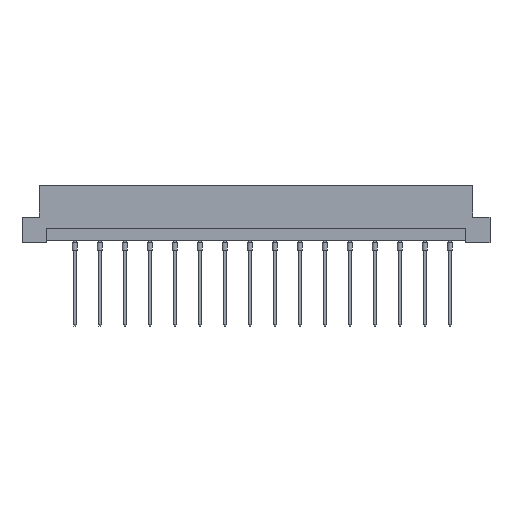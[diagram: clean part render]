
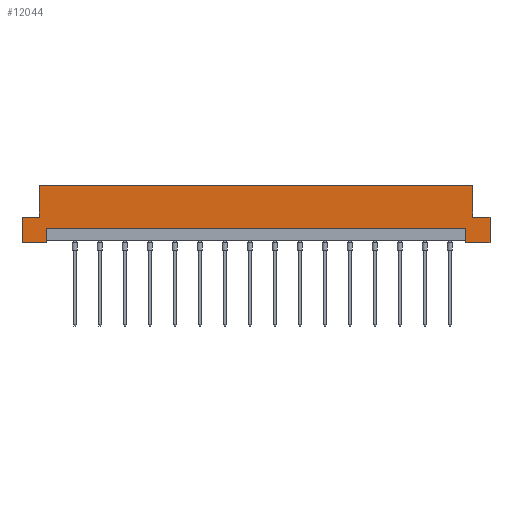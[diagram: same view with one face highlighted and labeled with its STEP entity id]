
A CAD part, front view. The second image highlights one B-rep face of the part: STEP entity #12044.
In plain terms, the highlighted planar face has unit normal (0, -1, 0).
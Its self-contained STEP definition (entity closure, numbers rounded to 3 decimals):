
#254 = LINE ( 'NONE', #3026, #791 ) ;
#526 = EDGE_CURVE ( 'NONE', #8135, #6141, #4010, .T. ) ;
#589 = CARTESIAN_POINT ( 'NONE',  ( -47.5, 0., 5.2 ) ) ;
#791 = VECTOR ( 'NONE', #2764, 1000. ) ;
#903 = LINE ( 'NONE', #14493, #12254 ) ;
#1053 = VECTOR ( 'NONE', #10106, 1000. ) ;
#1087 = VECTOR ( 'NONE', #8696, 1000. ) ;
#1603 = FACE_OUTER_BOUND ( 'NONE', #7244, .T. ) ;
#1693 = DIRECTION ( 'NONE',  ( 0., 1., 0. ) ) ;
#1768 = DIRECTION ( 'NONE',  ( 0., 0., 1. ) ) ;
#1848 = ORIENTED_EDGE ( 'NONE', *, *, #2364, .F. ) ;
#2083 = ORIENTED_EDGE ( 'NONE', *, *, #16746, .T. ) ;
#2117 = VERTEX_POINT ( 'NONE', #13574 ) ;
#2306 = CARTESIAN_POINT ( 'NONE',  ( 47.5, 0., 5.2 ) ) ;
#2364 = EDGE_CURVE ( 'NONE', #9708, #5236, #4027, .T. ) ;
#2464 = CARTESIAN_POINT ( 'NONE',  ( -47.5, 0., 0. ) ) ;
#2494 = VECTOR ( 'NONE', #13591, 1000. ) ;
#2764 = DIRECTION ( 'NONE',  ( -1., 0., 0. ) ) ;
#2993 = DIRECTION ( 'NONE',  ( -1., 0., 0. ) ) ;
#3026 = CARTESIAN_POINT ( 'NONE',  ( 42.6, 0., 2.9 ) ) ;
#3185 = CARTESIAN_POINT ( 'NONE',  ( -44., 0., 11.6 ) ) ;
#3362 = LINE ( 'NONE', #589, #1053 ) ;
#3499 = VERTEX_POINT ( 'NONE', #12302 ) ;
#3605 = EDGE_CURVE ( 'NONE', #7947, #10979, #9857, .T. ) ;
#3827 = VERTEX_POINT ( 'NONE', #9080 ) ;
#3889 = ORIENTED_EDGE ( 'NONE', *, *, #5770, .F. ) ;
#3934 = CARTESIAN_POINT ( 'NONE',  ( -44., 0., 5.2 ) ) ;
#3948 = DIRECTION ( 'NONE',  ( 0., 0., 1. ) ) ;
#4010 = LINE ( 'NONE', #9472, #17035 ) ;
#4027 = LINE ( 'NONE', #2464, #13573 ) ;
#4116 = ORIENTED_EDGE ( 'NONE', *, *, #3605, .F. ) ;
#4282 = CARTESIAN_POINT ( 'NONE',  ( 42.6, 0., 2.9 ) ) ;
#4294 = PLANE ( 'NONE',  #6593 ) ;
#4607 = VERTEX_POINT ( 'NONE', #7876 ) ;
#4753 = DIRECTION ( 'NONE',  ( 0., 0., 1. ) ) ;
#4862 = VECTOR ( 'NONE', #4753, 1000. ) ;
#5236 = VERTEX_POINT ( 'NONE', #9432 ) ;
#5342 = LINE ( 'NONE', #2306, #16268 ) ;
#5584 = ORIENTED_EDGE ( 'NONE', *, *, #7780, .F. ) ;
#5752 = VECTOR ( 'NONE', #13135, 1000. ) ;
#5770 = EDGE_CURVE ( 'NONE', #7161, #11679, #8915, .T. ) ;
#6141 = VERTEX_POINT ( 'NONE', #16254 ) ;
#6461 = CARTESIAN_POINT ( 'NONE',  ( -42.6, 0., 2.9 ) ) ;
#6593 = AXIS2_PLACEMENT_3D ( 'NONE', #13557, #1693, #1768 ) ;
#6619 = VECTOR ( 'NONE', #16775, 1000. ) ;
#6741 = VECTOR ( 'NONE', #2993, 1000. ) ;
#6823 = ORIENTED_EDGE ( 'NONE', *, *, #11260, .F. ) ;
#7161 = VERTEX_POINT ( 'NONE', #6461 ) ;
#7244 = EDGE_LOOP ( 'NONE', ( #14035, #13703, #5584, #14961, #6823, #2083, #13695, #4116, #14685, #1848, #13256, #3889 ) ) ;
#7431 = CARTESIAN_POINT ( 'NONE',  ( -42.6, 0., 0.5 ) ) ;
#7780 = EDGE_CURVE ( 'NONE', #4607, #6141, #12272, .T. ) ;
#7876 = CARTESIAN_POINT ( 'NONE',  ( 47.5, 0., 0. ) ) ;
#7947 = VERTEX_POINT ( 'NONE', #3934 ) ;
#8135 = VERTEX_POINT ( 'NONE', #4282 ) ;
#8140 = LINE ( 'NONE', #11959, #2494 ) ;
#8696 = DIRECTION ( 'NONE',  ( 1., 0., 0. ) ) ;
#8915 = LINE ( 'NONE', #7431, #6619 ) ;
#9080 = CARTESIAN_POINT ( 'NONE',  ( 47.5, 0., 5.2 ) ) ;
#9081 = LINE ( 'NONE', #13057, #5752 ) ;
#9215 = EDGE_CURVE ( 'NONE', #10979, #2117, #12779, .T. ) ;
#9291 = DIRECTION ( 'NONE',  ( 0., 0., -1. ) ) ;
#9432 = CARTESIAN_POINT ( 'NONE',  ( -47.5, 0., 5.2 ) ) ;
#9472 = CARTESIAN_POINT ( 'NONE',  ( 42.6, 0., 0.5 ) ) ;
#9631 = EDGE_CURVE ( 'NONE', #8135, #7161, #254, .T. ) ;
#9708 = VERTEX_POINT ( 'NONE', #10747 ) ;
#9848 = EDGE_CURVE ( 'NONE', #5236, #7947, #3362, .T. ) ;
#9857 = LINE ( 'NONE', #16609, #4862 ) ;
#10106 = DIRECTION ( 'NONE',  ( 1., 0., 0. ) ) ;
#10369 = DIRECTION ( 'NONE',  ( 1., 0., 0. ) ) ;
#10747 = CARTESIAN_POINT ( 'NONE',  ( -47.5, 0., 0. ) ) ;
#10979 = VERTEX_POINT ( 'NONE', #3185 ) ;
#11260 = EDGE_CURVE ( 'NONE', #3499, #3827, #5342, .T. ) ;
#11298 = EDGE_CURVE ( 'NONE', #3827, #4607, #9081, .T. ) ;
#11483 = CARTESIAN_POINT ( 'NONE',  ( -47.5, 0., 11.6 ) ) ;
#11679 = VERTEX_POINT ( 'NONE', #12535 ) ;
#11959 = CARTESIAN_POINT ( 'NONE',  ( -47.5, 0., 0. ) ) ;
#12044 = ADVANCED_FACE ( 'NONE', ( #1603 ), #4294, .F. ) ;
#12254 = VECTOR ( 'NONE', #14153, 1000. ) ;
#12272 = LINE ( 'NONE', #14851, #6741 ) ;
#12302 = CARTESIAN_POINT ( 'NONE',  ( 44., 0., 5.2 ) ) ;
#12535 = CARTESIAN_POINT ( 'NONE',  ( -42.6, 0., 0. ) ) ;
#12779 = LINE ( 'NONE', #11483, #1087 ) ;
#13057 = CARTESIAN_POINT ( 'NONE',  ( 47.5, 0., 0. ) ) ;
#13135 = DIRECTION ( 'NONE',  ( 0., 0., -1. ) ) ;
#13256 = ORIENTED_EDGE ( 'NONE', *, *, #14682, .F. ) ;
#13557 = CARTESIAN_POINT ( 'NONE',  ( -47.5, 0., 11.6 ) ) ;
#13573 = VECTOR ( 'NONE', #3948, 1000. ) ;
#13574 = CARTESIAN_POINT ( 'NONE',  ( 44., 0., 11.6 ) ) ;
#13591 = DIRECTION ( 'NONE',  ( -1., 0., 0. ) ) ;
#13695 = ORIENTED_EDGE ( 'NONE', *, *, #9215, .F. ) ;
#13703 = ORIENTED_EDGE ( 'NONE', *, *, #526, .T. ) ;
#14035 = ORIENTED_EDGE ( 'NONE', *, *, #9631, .F. ) ;
#14153 = DIRECTION ( 'NONE',  ( 0., 0., 1. ) ) ;
#14493 = CARTESIAN_POINT ( 'NONE',  ( 44., 0., 5.2 ) ) ;
#14682 = EDGE_CURVE ( 'NONE', #11679, #9708, #8140, .T. ) ;
#14685 = ORIENTED_EDGE ( 'NONE', *, *, #9848, .F. ) ;
#14851 = CARTESIAN_POINT ( 'NONE',  ( -47.5, 0., 0. ) ) ;
#14961 = ORIENTED_EDGE ( 'NONE', *, *, #11298, .F. ) ;
#16254 = CARTESIAN_POINT ( 'NONE',  ( 42.6, 0., 0. ) ) ;
#16268 = VECTOR ( 'NONE', #10369, 1000. ) ;
#16609 = CARTESIAN_POINT ( 'NONE',  ( -44., 0., 5.2 ) ) ;
#16746 = EDGE_CURVE ( 'NONE', #3499, #2117, #903, .T. ) ;
#16775 = DIRECTION ( 'NONE',  ( 0., 0., -1. ) ) ;
#17035 = VECTOR ( 'NONE', #9291, 1000. ) ;
